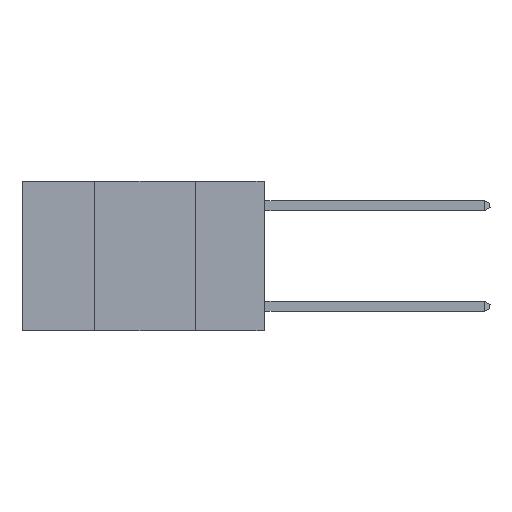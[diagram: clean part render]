
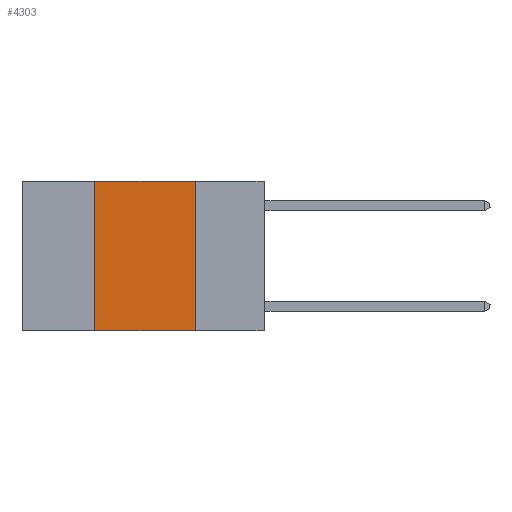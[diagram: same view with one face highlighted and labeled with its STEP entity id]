
A CAD part, left-side view. The second image highlights one B-rep face of the part: STEP entity #4303.
In plain terms, the highlighted planar face has unit normal (-1, 0, 0).
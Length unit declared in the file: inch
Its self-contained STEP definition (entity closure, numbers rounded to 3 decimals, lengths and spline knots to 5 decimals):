
#25 = LINE ( 'NONE', #2984, #5603 ) ;
#525 = VECTOR ( 'NONE', #12729, 39.37008 ) ;
#667 = CARTESIAN_POINT ( 'NONE',  ( 0., 0.17, 0. ) ) ;
#979 = EDGE_CURVE ( 'NONE', #7121, #7306, #10735, .T. ) ;
#1381 = ORIENTED_EDGE ( 'NONE', *, *, #1895, .T. ) ;
#1390 = DIRECTION ( 'NONE',  ( 0., 0., 1. ) ) ;
#1895 = EDGE_CURVE ( 'NONE', #7121, #12266, #7576, .T. ) ;
#2057 = ORIENTED_EDGE ( 'NONE', *, *, #979, .F. ) ;
#2984 = CARTESIAN_POINT ( 'NONE',  ( 0., 0.6, 0. ) ) ;
#3212 = VECTOR ( 'NONE', #1390, 39.37008 ) ;
#3543 = CARTESIAN_POINT ( 'NONE',  ( 0., 0.42, 0. ) ) ;
#3565 = EDGE_LOOP ( 'NONE', ( #14447, #11743, #2057, #1381 ) ) ;
#4303 = ADVANCED_FACE ( 'NONE', ( #11602 ), #5241, .F. ) ;
#5241 = PLANE ( 'NONE',  #14031 ) ;
#5446 = EDGE_CURVE ( 'NONE', #7688, #12266, #12373, .T. ) ;
#5603 = VECTOR ( 'NONE', #14179, 39.37008 ) ;
#6161 = CARTESIAN_POINT ( 'NONE',  ( 0., 0.6, 0. ) ) ;
#6264 = VECTOR ( 'NONE', #8425, 39.37008 ) ;
#7121 = VERTEX_POINT ( 'NONE', #9040 ) ;
#7306 = VERTEX_POINT ( 'NONE', #3543 ) ;
#7576 = LINE ( 'NONE', #11359, #525 ) ;
#7688 = VERTEX_POINT ( 'NONE', #12506 ) ;
#7791 = CARTESIAN_POINT ( 'NONE',  ( 0., 0.42, 0. ) ) ;
#8425 = DIRECTION ( 'NONE',  ( 0., 0., -1. ) ) ;
#9040 = CARTESIAN_POINT ( 'NONE',  ( 0., 0.42, -0.37 ) ) ;
#9071 = EDGE_CURVE ( 'NONE', #7306, #7688, #25, .T. ) ;
#10118 = DIRECTION ( 'NONE',  ( 1., 0., 0. ) ) ;
#10238 = CARTESIAN_POINT ( 'NONE',  ( 0., 0.17, -0.37 ) ) ;
#10735 = LINE ( 'NONE', #7791, #3212 ) ;
#11359 = CARTESIAN_POINT ( 'NONE',  ( 0., 0.6, -0.37 ) ) ;
#11602 = FACE_OUTER_BOUND ( 'NONE', #3565, .T. ) ;
#11743 = ORIENTED_EDGE ( 'NONE', *, *, #9071, .F. ) ;
#12266 = VERTEX_POINT ( 'NONE', #10238 ) ;
#12373 = LINE ( 'NONE', #667, #6264 ) ;
#12506 = CARTESIAN_POINT ( 'NONE',  ( 0., 0.17, 0. ) ) ;
#12729 = DIRECTION ( 'NONE',  ( 0., -1., 0. ) ) ;
#14031 = AXIS2_PLACEMENT_3D ( 'NONE', #6161, #10118, #15466 ) ;
#14179 = DIRECTION ( 'NONE',  ( 0., -1., 0. ) ) ;
#14447 = ORIENTED_EDGE ( 'NONE', *, *, #5446, .F. ) ;
#15466 = DIRECTION ( 'NONE',  ( 0., 0., -1. ) ) ;
